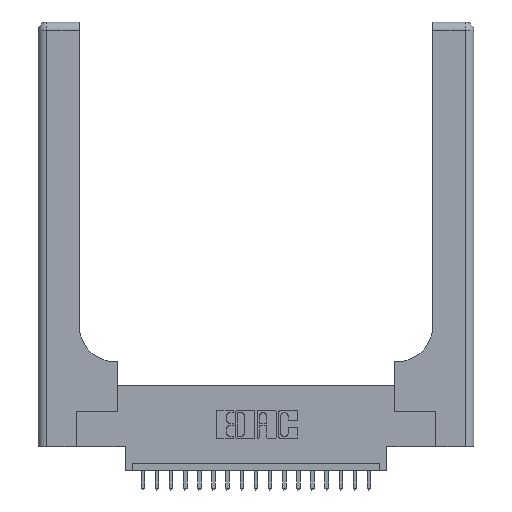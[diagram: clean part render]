
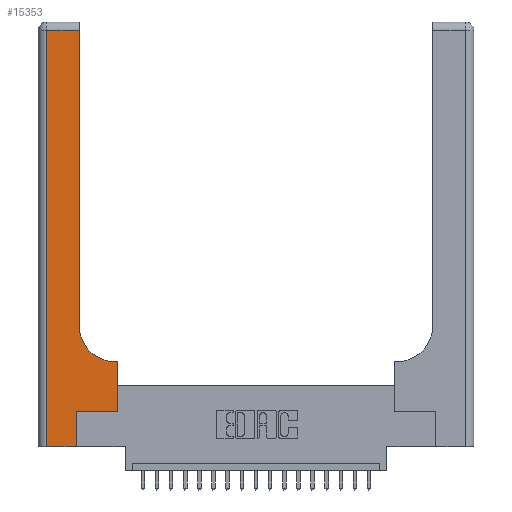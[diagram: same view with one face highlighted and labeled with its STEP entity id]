
A CAD part, top view. The second image highlights one B-rep face of the part: STEP entity #15353.
In plain terms, the highlighted planar face has unit normal (0, 0, 1).
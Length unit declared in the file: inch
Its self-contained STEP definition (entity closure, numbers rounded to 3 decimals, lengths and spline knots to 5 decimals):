
#391 = LINE ( 'NONE', #12657, #5589 ) ;
#558 = ORIENTED_EDGE ( 'NONE', *, *, #7199, .T. ) ;
#1062 = DIRECTION ( 'NONE',  ( -1., 0., 0. ) ) ;
#1139 = VERTEX_POINT ( 'NONE', #5665 ) ;
#1505 = EDGE_CURVE ( 'NONE', #1899, #1139, #2726, .T. ) ;
#1899 = VERTEX_POINT ( 'NONE', #20317 ) ;
#1996 = VECTOR ( 'NONE', #18258, 39.37008 ) ;
#2345 = VERTEX_POINT ( 'NONE', #2395 ) ;
#2356 = AXIS2_PLACEMENT_3D ( 'NONE', #18016, #13362, #13146 ) ;
#2372 = CARTESIAN_POINT ( 'NONE',  ( 0., 2.94, 0.37 ) ) ;
#2395 = CARTESIAN_POINT ( 'NONE',  ( 0.2915, 0.85, 0.37 ) ) ;
#2502 = CARTESIAN_POINT ( 'NONE',  ( 0., 3., 0.37 ) ) ;
#2726 = LINE ( 'NONE', #7410, #19849 ) ;
#2731 = EDGE_CURVE ( 'NONE', #4078, #2345, #6054, .T. ) ;
#3063 = CARTESIAN_POINT ( 'NONE',  ( 0.5585, 0.25, 0.37 ) ) ;
#3709 = DIRECTION ( 'NONE',  ( 0., 1., 0. ) ) ;
#3876 = CARTESIAN_POINT ( 'NONE',  ( 0.06, 0., 0.37 ) ) ;
#3925 = LINE ( 'NONE', #2372, #17646 ) ;
#4078 = VERTEX_POINT ( 'NONE', #10483 ) ;
#4379 = ORIENTED_EDGE ( 'NONE', *, *, #13189, .T. ) ;
#4513 = CARTESIAN_POINT ( 'NONE',  ( 0.06, 3., 0.37 ) ) ;
#5589 = VECTOR ( 'NONE', #9301, 39.37008 ) ;
#5665 = CARTESIAN_POINT ( 'NONE',  ( 0.269, 0.25, 0.37 ) ) ;
#5690 = ORIENTED_EDGE ( 'NONE', *, *, #6172, .T. ) ;
#5771 = EDGE_LOOP ( 'NONE', ( #5902, #11662, #5690, #18774, #20543, #558, #4379, #9300, #13249 ) ) ;
#5832 = VERTEX_POINT ( 'NONE', #8138 ) ;
#5902 = ORIENTED_EDGE ( 'NONE', *, *, #7328, .T. ) ;
#5935 = DIRECTION ( 'NONE',  ( -1., 0., 0. ) ) ;
#6054 = CIRCLE ( 'NONE', #2356, 0.25 ) ;
#6172 = EDGE_CURVE ( 'NONE', #9739, #14735, #10055, .T. ) ;
#6636 = VECTOR ( 'NONE', #3709, 39.37008 ) ;
#7199 = EDGE_CURVE ( 'NONE', #1139, #10034, #391, .T. ) ;
#7328 = EDGE_CURVE ( 'NONE', #2345, #20390, #20908, .T. ) ;
#7410 = CARTESIAN_POINT ( 'NONE',  ( 0.269, 0., 0.37 ) ) ;
#8138 = CARTESIAN_POINT ( 'NONE',  ( 0.5585, 0.6, 0.37 ) ) ;
#8371 = DIRECTION ( 'NONE',  ( 1., 0., 0. ) ) ;
#8627 = VECTOR ( 'NONE', #19697, 39.37008 ) ;
#8669 = CARTESIAN_POINT ( 'NONE',  ( 0.06, 2.94, 0.37 ) ) ;
#8693 = VECTOR ( 'NONE', #5935, 39.37008 ) ;
#9300 = ORIENTED_EDGE ( 'NONE', *, *, #19592, .T. ) ;
#9301 = DIRECTION ( 'NONE',  ( 1., 0., 0. ) ) ;
#9739 = VERTEX_POINT ( 'NONE', #8669 ) ;
#10034 = VERTEX_POINT ( 'NONE', #3063 ) ;
#10040 = EDGE_CURVE ( 'NONE', #20390, #9739, #3925, .T. ) ;
#10055 = LINE ( 'NONE', #4513, #1996 ) ;
#10124 = AXIS2_PLACEMENT_3D ( 'NONE', #2502, #15881, #1062 ) ;
#10483 = CARTESIAN_POINT ( 'NONE',  ( 0.5415, 0.6, 0.37 ) ) ;
#10577 = FACE_OUTER_BOUND ( 'NONE', #5771, .T. ) ;
#11662 = ORIENTED_EDGE ( 'NONE', *, *, #10040, .T. ) ;
#12322 = LINE ( 'NONE', #21521, #18826 ) ;
#12657 = CARTESIAN_POINT ( 'NONE',  ( 0.269, 0.25, 0.37 ) ) ;
#13146 = DIRECTION ( 'NONE',  ( 1., 0., 0. ) ) ;
#13189 = EDGE_CURVE ( 'NONE', #10034, #5832, #16350, .T. ) ;
#13249 = ORIENTED_EDGE ( 'NONE', *, *, #2731, .T. ) ;
#13354 = DIRECTION ( 'NONE',  ( 0., 1., 0. ) ) ;
#13362 = DIRECTION ( 'NONE',  ( 0., 0., -1. ) ) ;
#13617 = DIRECTION ( 'NONE',  ( -1., 0., 0. ) ) ;
#14300 = CARTESIAN_POINT ( 'NONE',  ( 0.2915, 0.6, 0.37 ) ) ;
#14350 = PLANE ( 'NONE',  #10124 ) ;
#14521 = CARTESIAN_POINT ( 'NONE',  ( 0.5585, 0.25, 0.37 ) ) ;
#14735 = VERTEX_POINT ( 'NONE', #3876 ) ;
#15353 = ADVANCED_FACE ( 'NONE', ( #10577 ), #14350, .F. ) ;
#15881 = DIRECTION ( 'NONE',  ( 0., 0., -1. ) ) ;
#16350 = LINE ( 'NONE', #14521, #8627 ) ;
#16442 = EDGE_CURVE ( 'NONE', #14735, #1899, #12322, .T. ) ;
#16878 = CARTESIAN_POINT ( 'NONE',  ( 0.2915, 2.94, 0.37 ) ) ;
#17201 = LINE ( 'NONE', #14300, #8693 ) ;
#17646 = VECTOR ( 'NONE', #13617, 39.37008 ) ;
#18016 = CARTESIAN_POINT ( 'NONE',  ( 0.5415, 0.85, 0.37 ) ) ;
#18258 = DIRECTION ( 'NONE',  ( 0., -1., 0. ) ) ;
#18647 = CARTESIAN_POINT ( 'NONE',  ( 0.2915, 3., 0.37 ) ) ;
#18774 = ORIENTED_EDGE ( 'NONE', *, *, #16442, .T. ) ;
#18826 = VECTOR ( 'NONE', #8371, 39.37008 ) ;
#19592 = EDGE_CURVE ( 'NONE', #5832, #4078, #17201, .T. ) ;
#19697 = DIRECTION ( 'NONE',  ( 0., 1., 0. ) ) ;
#19849 = VECTOR ( 'NONE', #13354, 39.37008 ) ;
#20317 = CARTESIAN_POINT ( 'NONE',  ( 0.269, 0., 0.37 ) ) ;
#20390 = VERTEX_POINT ( 'NONE', #16878 ) ;
#20543 = ORIENTED_EDGE ( 'NONE', *, *, #1505, .T. ) ;
#20908 = LINE ( 'NONE', #18647, #6636 ) ;
#21521 = CARTESIAN_POINT ( 'NONE',  ( 0., 0., 0.37 ) ) ;
